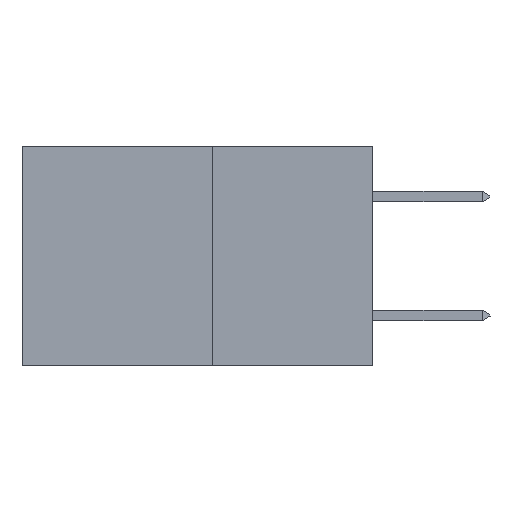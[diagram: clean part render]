
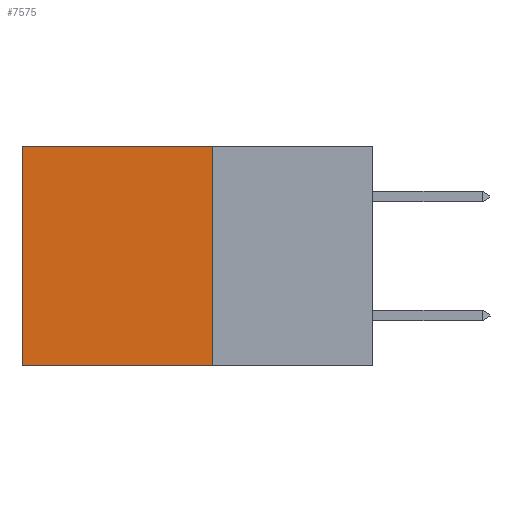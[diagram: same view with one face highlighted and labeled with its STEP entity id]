
A CAD part, left-side view. The second image highlights one B-rep face of the part: STEP entity #7575.
In plain terms, the highlighted planar face has unit normal (-1, 0, 0).
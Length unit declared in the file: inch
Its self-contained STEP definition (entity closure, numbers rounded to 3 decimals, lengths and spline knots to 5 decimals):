
#147 = DIRECTION ( 'NONE',  ( 0., 1., 0. ) ) ;
#438 = CARTESIAN_POINT ( 'NONE',  ( 0.277, 0.27, 0. ) ) ;
#552 = CARTESIAN_POINT ( 'NONE',  ( 0.277, 0.27, -0.37 ) ) ;
#760 = EDGE_LOOP ( 'NONE', ( #8770, #8571, #8177, #3969 ) ) ;
#1029 = VECTOR ( 'NONE', #6955, 39.37008 ) ;
#1304 = LINE ( 'NONE', #5561, #1029 ) ;
#1861 = CARTESIAN_POINT ( 'NONE',  ( 0.277, 0.27, -0.37 ) ) ;
#1995 = FACE_OUTER_BOUND ( 'NONE', #760, .T. ) ;
#2132 = CARTESIAN_POINT ( 'NONE',  ( 0.277, 0.27, 0. ) ) ;
#2571 = EDGE_CURVE ( 'NONE', #6947, #4319, #1304, .T. ) ;
#2659 = DIRECTION ( 'NONE',  ( 1., 0., 0. ) ) ;
#2943 = CARTESIAN_POINT ( 'NONE',  ( 0.277, 0.59, -0.37 ) ) ;
#3160 = VECTOR ( 'NONE', #4648, 39.37008 ) ;
#3357 = VERTEX_POINT ( 'NONE', #3921 ) ;
#3921 = CARTESIAN_POINT ( 'NONE',  ( 0.277, 0.59, 0. ) ) ;
#3969 = ORIENTED_EDGE ( 'NONE', *, *, #4589, .T. ) ;
#4004 = VECTOR ( 'NONE', #147, 39.37008 ) ;
#4319 = VERTEX_POINT ( 'NONE', #2943 ) ;
#4466 = CARTESIAN_POINT ( 'NONE',  ( 0.277, 0.59, -0.37 ) ) ;
#4589 = EDGE_CURVE ( 'NONE', #7090, #3357, #6304, .T. ) ;
#4648 = DIRECTION ( 'NONE',  ( 0., 0., -1. ) ) ;
#4654 = DIRECTION ( 'NONE',  ( 0., 0., -1. ) ) ;
#4904 = EDGE_CURVE ( 'NONE', #3357, #4319, #5013, .T. ) ;
#5013 = LINE ( 'NONE', #4466, #3160 ) ;
#5234 = VECTOR ( 'NONE', #4654, 39.37008 ) ;
#5329 = AXIS2_PLACEMENT_3D ( 'NONE', #1861, #2659, #8018 ) ;
#5561 = CARTESIAN_POINT ( 'NONE',  ( 0.277, 0.27, -0.37 ) ) ;
#6304 = LINE ( 'NONE', #438, #4004 ) ;
#6947 = VERTEX_POINT ( 'NONE', #9503 ) ;
#6955 = DIRECTION ( 'NONE',  ( 0., 1., 0. ) ) ;
#7090 = VERTEX_POINT ( 'NONE', #2132 ) ;
#7214 = EDGE_CURVE ( 'NONE', #7090, #6947, #9328, .T. ) ;
#7287 = PLANE ( 'NONE',  #5329 ) ;
#7575 = ADVANCED_FACE ( 'NONE', ( #1995 ), #7287, .F. ) ;
#8018 = DIRECTION ( 'NONE',  ( 0., 0., -1. ) ) ;
#8177 = ORIENTED_EDGE ( 'NONE', *, *, #7214, .F. ) ;
#8571 = ORIENTED_EDGE ( 'NONE', *, *, #2571, .F. ) ;
#8770 = ORIENTED_EDGE ( 'NONE', *, *, #4904, .T. ) ;
#9328 = LINE ( 'NONE', #552, #5234 ) ;
#9503 = CARTESIAN_POINT ( 'NONE',  ( 0.277, 0.27, -0.37 ) ) ;
